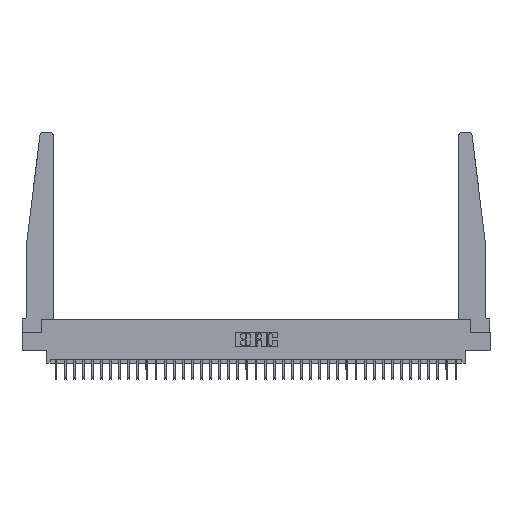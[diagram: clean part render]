
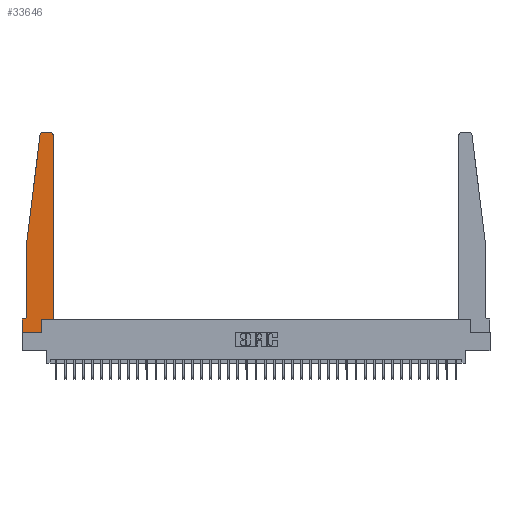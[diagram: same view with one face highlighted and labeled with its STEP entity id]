
A CAD part, top view. The second image highlights one B-rep face of the part: STEP entity #33646.
In plain terms, the highlighted planar face has unit normal (0, 0, 1).
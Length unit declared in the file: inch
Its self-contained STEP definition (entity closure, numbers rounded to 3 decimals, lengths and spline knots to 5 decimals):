
#3 = ORIENTED_EDGE ( 'NONE', *, *, #12019, .T. ) ;
#47 = LINE ( 'NONE', #2328, #21226 ) ;
#196 = EDGE_CURVE ( 'NONE', #16707, #23056, #13627, .T. ) ;
#481 = ORIENTED_EDGE ( 'NONE', *, *, #17884, .T. ) ;
#1390 = CARTESIAN_POINT ( 'NONE',  ( 0., 0.1875, 0.37 ) ) ;
#1864 = ORIENTED_EDGE ( 'NONE', *, *, #196, .T. ) ;
#1917 = DIRECTION ( 'NONE',  ( 1., 0., 0. ) ) ;
#2328 = CARTESIAN_POINT ( 'NONE',  ( 0.065, 1.25, 0.37 ) ) ;
#2890 = DIRECTION ( 'NONE',  ( 0., 1., 0. ) ) ;
#3048 = CARTESIAN_POINT ( 'NONE',  ( 0.065, 1.25, 0.37 ) ) ;
#3130 = EDGE_LOOP ( 'NONE', ( #24520, #5807, #3, #26609, #30163, #22060, #10606, #19438, #481, #24342, #1864, #34839 ) ) ;
#3609 = CARTESIAN_POINT ( 'NONE',  ( 0.065, 1.25, 0.37 ) ) ;
#4521 = CARTESIAN_POINT ( 'NONE',  ( 0.425, 0.18, 0.37 ) ) ;
#4759 = AXIS2_PLACEMENT_3D ( 'NONE', #29930, #13227, #32456 ) ;
#4863 = DIRECTION ( 'NONE',  ( -1., 0., 0. ) ) ;
#5055 = DIRECTION ( 'NONE',  ( 0., 0., 1. ) ) ;
#5124 = CARTESIAN_POINT ( 'NONE',  ( 0.27653, 2.75, 0.37 ) ) ;
#5807 = ORIENTED_EDGE ( 'NONE', *, *, #19983, .T. ) ;
#5873 = DIRECTION ( 'NONE',  ( 0., -1., 0. ) ) ;
#5962 = VERTEX_POINT ( 'NONE', #1390 ) ;
#6002 = DIRECTION ( 'NONE',  ( 0., 0., -1. ) ) ;
#7514 = DIRECTION ( 'NONE',  ( 1., 0., 0. ) ) ;
#7767 = CARTESIAN_POINT ( 'NONE',  ( 0.425, 0.18, 0.37 ) ) ;
#7829 = VECTOR ( 'NONE', #20711, 39.37008 ) ;
#7965 = EDGE_CURVE ( 'NONE', #22505, #16330, #11566, .T. ) ;
#8044 = CARTESIAN_POINT ( 'NONE',  ( 0.425, 2.72, 0.37 ) ) ;
#9579 = LINE ( 'NONE', #32861, #7829 ) ;
#10115 = DIRECTION ( 'NONE',  ( 0., 1., 0. ) ) ;
#10606 = ORIENTED_EDGE ( 'NONE', *, *, #21403, .T. ) ;
#11281 = CIRCLE ( 'NONE', #28608, 0.05 ) ;
#11285 = VERTEX_POINT ( 'NONE', #21895 ) ;
#11566 = LINE ( 'NONE', #3048, #17170 ) ;
#11732 = VERTEX_POINT ( 'NONE', #14323 ) ;
#11889 = VECTOR ( 'NONE', #4863, 39.37008 ) ;
#12019 = EDGE_CURVE ( 'NONE', #33576, #22505, #47, .T. ) ;
#12488 = LINE ( 'NONE', #14068, #15941 ) ;
#12980 = AXIS2_PLACEMENT_3D ( 'NONE', #26973, #5055, #1917 ) ;
#13182 = EDGE_CURVE ( 'NONE', #11732, #26495, #15694, .T. ) ;
#13227 = DIRECTION ( 'NONE',  ( 0., 0., 1. ) ) ;
#13627 = LINE ( 'NONE', #7767, #20516 ) ;
#14068 = CARTESIAN_POINT ( 'NONE',  ( 0., 0., 0.37 ) ) ;
#14264 = EDGE_CURVE ( 'NONE', #16330, #15205, #11281, .T. ) ;
#14323 = CARTESIAN_POINT ( 'NONE',  ( 0., 0., 0.37 ) ) ;
#14962 = CARTESIAN_POINT ( 'NONE',  ( 0.2605, 0.18, 0.37 ) ) ;
#15090 = CARTESIAN_POINT ( 'NONE',  ( 0.065, 0.1875, 0.37 ) ) ;
#15170 = FACE_OUTER_BOUND ( 'NONE', #3130, .T. ) ;
#15205 = VERTEX_POINT ( 'NONE', #24319 ) ;
#15694 = LINE ( 'NONE', #22027, #25577 ) ;
#15941 = VECTOR ( 'NONE', #5873, 39.37008 ) ;
#16330 = VERTEX_POINT ( 'NONE', #20255 ) ;
#16429 = VERTEX_POINT ( 'NONE', #14962 ) ;
#16707 = VERTEX_POINT ( 'NONE', #4521 ) ;
#16799 = VERTEX_POINT ( 'NONE', #5124 ) ;
#17170 = VECTOR ( 'NONE', #27906, 39.37008 ) ;
#17884 = EDGE_CURVE ( 'NONE', #26495, #16429, #24846, .T. ) ;
#17892 = DIRECTION ( 'NONE',  ( 0., 0., 1. ) ) ;
#18316 = DIRECTION ( 'NONE',  ( -1., 0., 0. ) ) ;
#18499 = EDGE_CURVE ( 'NONE', #11285, #16799, #19206, .T. ) ;
#19206 = LINE ( 'NONE', #35313, #11889 ) ;
#19438 = ORIENTED_EDGE ( 'NONE', *, *, #13182, .T. ) ;
#19982 = DIRECTION ( 'NONE',  ( -1., 0., 0. ) ) ;
#19983 = EDGE_CURVE ( 'NONE', #16799, #33576, #31933, .T. ) ;
#20255 = CARTESIAN_POINT ( 'NONE',  ( 0.065, 0.2375, 0.37 ) ) ;
#20516 = VECTOR ( 'NONE', #2890, 39.37008 ) ;
#20711 = DIRECTION ( 'NONE',  ( 1., 0., 0. ) ) ;
#20958 = CARTESIAN_POINT ( 'NONE',  ( 0.015, 0.2375, 0.37 ) ) ;
#21226 = VECTOR ( 'NONE', #27407, 39.37008 ) ;
#21284 = VECTOR ( 'NONE', #18316, 39.37008 ) ;
#21403 = EDGE_CURVE ( 'NONE', #5962, #11732, #12488, .T. ) ;
#21895 = CARTESIAN_POINT ( 'NONE',  ( 0.395, 2.75, 0.37 ) ) ;
#22027 = CARTESIAN_POINT ( 'NONE',  ( 0., 0., 0.37 ) ) ;
#22060 = ORIENTED_EDGE ( 'NONE', *, *, #32644, .T. ) ;
#22505 = VERTEX_POINT ( 'NONE', #3609 ) ;
#22833 = CARTESIAN_POINT ( 'NONE',  ( 0.2605, 0., 0.37 ) ) ;
#23056 = VERTEX_POINT ( 'NONE', #8044 ) ;
#23874 = AXIS2_PLACEMENT_3D ( 'NONE', #32045, #17892, #7514 ) ;
#24319 = CARTESIAN_POINT ( 'NONE',  ( 0.015, 0.1875, 0.37 ) ) ;
#24342 = ORIENTED_EDGE ( 'NONE', *, *, #33817, .T. ) ;
#24520 = ORIENTED_EDGE ( 'NONE', *, *, #18499, .T. ) ;
#24781 = DIRECTION ( 'NONE',  ( 1., 0., 0. ) ) ;
#24846 = LINE ( 'NONE', #34128, #29154 ) ;
#25577 = VECTOR ( 'NONE', #24781, 39.37008 ) ;
#26495 = VERTEX_POINT ( 'NONE', #22833 ) ;
#26609 = ORIENTED_EDGE ( 'NONE', *, *, #7965, .T. ) ;
#26732 = CARTESIAN_POINT ( 'NONE',  ( 0.24675, 2.72367, 0.37 ) ) ;
#26973 = CARTESIAN_POINT ( 'NONE',  ( 0., 0.1875, 0.37 ) ) ;
#27407 = DIRECTION ( 'NONE',  ( -0.122, -0.992, 0. ) ) ;
#27906 = DIRECTION ( 'NONE',  ( 0., -1., 0. ) ) ;
#28584 = EDGE_CURVE ( 'NONE', #23056, #11285, #30124, .T. ) ;
#28608 = AXIS2_PLACEMENT_3D ( 'NONE', #20958, #6002, #19982 ) ;
#29154 = VECTOR ( 'NONE', #10115, 39.37008 ) ;
#29441 = LINE ( 'NONE', #15090, #21284 ) ;
#29930 = CARTESIAN_POINT ( 'NONE',  ( 0.395, 2.72, 0.37 ) ) ;
#30124 = CIRCLE ( 'NONE', #4759, 0.03 ) ;
#30163 = ORIENTED_EDGE ( 'NONE', *, *, #14264, .T. ) ;
#31933 = CIRCLE ( 'NONE', #23874, 0.03 ) ;
#32045 = CARTESIAN_POINT ( 'NONE',  ( 0.27653, 2.72, 0.37 ) ) ;
#32456 = DIRECTION ( 'NONE',  ( 1., 0., 0. ) ) ;
#32644 = EDGE_CURVE ( 'NONE', #15205, #5962, #29441, .T. ) ;
#32861 = CARTESIAN_POINT ( 'NONE',  ( 0.425, 0.18, 0.37 ) ) ;
#33576 = VERTEX_POINT ( 'NONE', #26732 ) ;
#33646 = ADVANCED_FACE ( 'NONE', ( #15170 ), #34914, .T. ) ;
#33817 = EDGE_CURVE ( 'NONE', #16429, #16707, #9579, .T. ) ;
#34128 = CARTESIAN_POINT ( 'NONE',  ( 0.2605, 0.18, 0.37 ) ) ;
#34839 = ORIENTED_EDGE ( 'NONE', *, *, #28584, .T. ) ;
#34914 = PLANE ( 'NONE',  #12980 ) ;
#35313 = CARTESIAN_POINT ( 'NONE',  ( 0.25, 2.75, 0.37 ) ) ;
